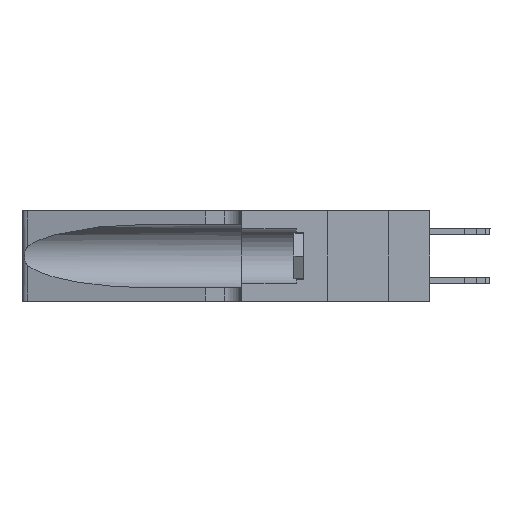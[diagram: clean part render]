
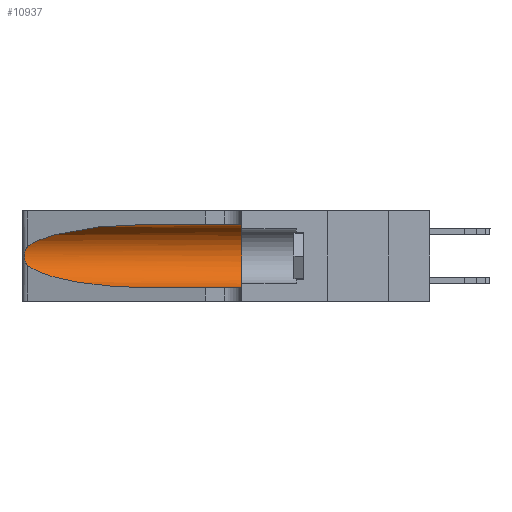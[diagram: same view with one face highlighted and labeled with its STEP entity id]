
A CAD part, left-side view. The second image highlights one B-rep face of the part: STEP entity #10937.
In plain terms, the highlighted cylindrical face has radius 3.308 mm (diameter 6.617 mm), a partial arc.
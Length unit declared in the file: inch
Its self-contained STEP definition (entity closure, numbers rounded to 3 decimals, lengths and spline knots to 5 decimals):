
#892 = CARTESIAN_POINT ( 'NONE',  ( 0.25555, 1.22993, 0.14849 ) ) ;
#899 = CYLINDRICAL_SURFACE ( 'NONE', #19962, 0.13025 ) ;
#1081 = EDGE_CURVE ( 'NONE', #21662, #8447, #6607, .T. ) ;
#1470 = CARTESIAN_POINT ( 'NONE',  ( 0.1305, 0.35, 0.185 ) ) ;
#1933 = CARTESIAN_POINT ( 'NONE',  ( 0.25487, 1.22718, 0.14631 ) ) ;
#2222 = CARTESIAN_POINT ( 'NONE',  ( 0.1305, 0.72297, 0.05475 ) ) ;
#2813 = CARTESIAN_POINT ( 'NONE',  ( 0.2373, 1.15595, 0.28018 ) ) ;
#2950 = CARTESIAN_POINT ( 'NONE',  ( 0.1305, 0.72297, 0.05475 ) ) ;
#3074 = CARTESIAN_POINT ( 'NONE',  ( 0.26075, 1.23896, 0.178 ) ) ;
#3097 = VERTEX_POINT ( 'NONE', #1933 ) ;
#3246 =( BOUNDED_CURVE ( )  B_SPLINE_CURVE ( 3, ( #10583, #22651, #9520, #2950 ),
 .UNSPECIFIED., .F., .F. ) 
 B_SPLINE_CURVE_WITH_KNOTS ( ( 4, 4 ),
 ( 3.44316, 4.71239 ),
 .UNSPECIFIED. ) 
 CURVE ( )  GEOMETRIC_REPRESENTATION_ITEM ( )  RATIONAL_B_SPLINE_CURVE ( ( 1., 0.87, 0.87, 1. ) ) 
 REPRESENTATION_ITEM ( '' )  );
#4076 = B_SPLINE_CURVE_WITH_KNOTS ( 'NONE', 3,
 ( #21431, #13268, #11193, #25805, #23622, #17405, #5046, #3074, #19617, #19441, #9105, #25632, #892, #15600 ),
 .UNSPECIFIED., .F., .F.,
 ( 4, 2, 2, 2, 2, 2, 4 ),
 ( 0., 0.00027, 0.00053, 0.00107, 0.0016, 0.00187, 0.00214 ),
 .UNSPECIFIED. ) ;
#4954 = CARTESIAN_POINT ( 'NONE',  ( 0.1305, 0.72297, 0.31525 ) ) ;
#5046 = CARTESIAN_POINT ( 'NONE',  ( 0.26075, 1.23896, 0.19203 ) ) ;
#5321 = CARTESIAN_POINT ( 'NONE',  ( 0.1305, 1.61858, 0.05475 ) ) ;
#6013 = ORIENTED_EDGE ( 'NONE', *, *, #6908, .T. ) ;
#6290 = DIRECTION ( 'NONE',  ( 0., -1., 0. ) ) ;
#6545 = ORIENTED_EDGE ( 'NONE', *, *, #19073, .T. ) ;
#6607 = LINE ( 'NONE', #24965, #24341 ) ;
#6908 = EDGE_CURVE ( 'NONE', #3097, #22408, #3246, .T. ) ;
#6916 = AXIS2_PLACEMENT_3D ( 'NONE', #1470, #24186, #9655 ) ;
#6939 = CARTESIAN_POINT ( 'NONE',  ( 0.18966, 0.96281, 0.31525 ) ) ;
#7199 = DIRECTION ( 'NONE',  ( 0., 0., -1. ) ) ;
#7292 = EDGE_LOOP ( 'NONE', ( #12172, #6545, #6013, #8333, #18867, #19686 ) ) ;
#7824 = LINE ( 'NONE', #5321, #22986 ) ;
#8333 = ORIENTED_EDGE ( 'NONE', *, *, #8410, .T. ) ;
#8410 = EDGE_CURVE ( 'NONE', #22408, #14646, #7824, .T. ) ;
#8447 = VERTEX_POINT ( 'NONE', #21984 ) ;
#8847 =( BOUNDED_CURVE ( )  B_SPLINE_CURVE ( 3, ( #4954, #6939, #2813, #23989 ),
 .UNSPECIFIED., .F., .F. ) 
 B_SPLINE_CURVE_WITH_KNOTS ( ( 4, 4 ),
 ( 1.5708, 2.84003 ),
 .UNSPECIFIED. ) 
 CURVE ( )  GEOMETRIC_REPRESENTATION_ITEM ( )  RATIONAL_B_SPLINE_CURVE ( ( 1., 0.87, 0.87, 1. ) ) 
 REPRESENTATION_ITEM ( '' )  );
#9105 = CARTESIAN_POINT ( 'NONE',  ( 0.25789, 1.23486, 0.15765 ) ) ;
#9520 = CARTESIAN_POINT ( 'NONE',  ( 0.18966, 0.96281, 0.05475 ) ) ;
#9655 = DIRECTION ( 'NONE',  ( 0., 0., 1. ) ) ;
#10583 = CARTESIAN_POINT ( 'NONE',  ( 0.25487, 1.22718, 0.14631 ) ) ;
#10733 = CIRCLE ( 'NONE', #6916, 0.13025 ) ;
#10937 = ADVANCED_FACE ( 'NONE', ( #19926 ), #899, .F. ) ;
#11193 = CARTESIAN_POINT ( 'NONE',  ( 0.25639, 1.23184, 0.21858 ) ) ;
#12172 = ORIENTED_EDGE ( 'NONE', *, *, #17105, .T. ) ;
#13268 = CARTESIAN_POINT ( 'NONE',  ( 0.25555, 1.22994, 0.2215 ) ) ;
#14377 = EDGE_CURVE ( 'NONE', #8447, #14646, #10733, .T. ) ;
#14646 = VERTEX_POINT ( 'NONE', #23071 ) ;
#15488 = CARTESIAN_POINT ( 'NONE',  ( 0.1305, 1.61858, 0.185 ) ) ;
#15600 = CARTESIAN_POINT ( 'NONE',  ( 0.25487, 1.22718, 0.14631 ) ) ;
#17105 = EDGE_CURVE ( 'NONE', #21662, #20255, #8847, .T. ) ;
#17405 = CARTESIAN_POINT ( 'NONE',  ( 0.26018, 1.23835, 0.19895 ) ) ;
#17687 = DIRECTION ( 'NONE',  ( 0., -1., 0. ) ) ;
#18867 = ORIENTED_EDGE ( 'NONE', *, *, #14377, .F. ) ;
#19073 = EDGE_CURVE ( 'NONE', #20255, #3097, #4076, .T. ) ;
#19441 = CARTESIAN_POINT ( 'NONE',  ( 0.25856, 1.23593, 0.16098 ) ) ;
#19607 = DIRECTION ( 'NONE',  ( 0., -1., 0. ) ) ;
#19617 = CARTESIAN_POINT ( 'NONE',  ( 0.26017, 1.23833, 0.17102 ) ) ;
#19686 = ORIENTED_EDGE ( 'NONE', *, *, #1081, .F. ) ;
#19926 = FACE_OUTER_BOUND ( 'NONE', #7292, .T. ) ;
#19962 = AXIS2_PLACEMENT_3D ( 'NONE', #15488, #19607, #7199 ) ;
#20255 = VERTEX_POINT ( 'NONE', #23109 ) ;
#21431 = CARTESIAN_POINT ( 'NONE',  ( 0.25487, 1.22718, 0.22369 ) ) ;
#21662 = VERTEX_POINT ( 'NONE', #23424 ) ;
#21984 = CARTESIAN_POINT ( 'NONE',  ( 0.1305, 0.35, 0.31525 ) ) ;
#22408 = VERTEX_POINT ( 'NONE', #2222 ) ;
#22651 = CARTESIAN_POINT ( 'NONE',  ( 0.2373, 1.15595, 0.08982 ) ) ;
#22986 = VECTOR ( 'NONE', #17687, 39.37008 ) ;
#23071 = CARTESIAN_POINT ( 'NONE',  ( 0.1305, 0.35, 0.05475 ) ) ;
#23109 = CARTESIAN_POINT ( 'NONE',  ( 0.25487, 1.22718, 0.22369 ) ) ;
#23424 = CARTESIAN_POINT ( 'NONE',  ( 0.1305, 0.72297, 0.31525 ) ) ;
#23622 = CARTESIAN_POINT ( 'NONE',  ( 0.25854, 1.2359, 0.20912 ) ) ;
#23989 = CARTESIAN_POINT ( 'NONE',  ( 0.25487, 1.22718, 0.22369 ) ) ;
#24186 = DIRECTION ( 'NONE',  ( 0., 1., 0. ) ) ;
#24341 = VECTOR ( 'NONE', #6290, 39.37008 ) ;
#24965 = CARTESIAN_POINT ( 'NONE',  ( 0.1305, 1.61858, 0.31525 ) ) ;
#25632 = CARTESIAN_POINT ( 'NONE',  ( 0.25639, 1.23186, 0.15144 ) ) ;
#25805 = CARTESIAN_POINT ( 'NONE',  ( 0.25787, 1.23484, 0.2124 ) ) ;
